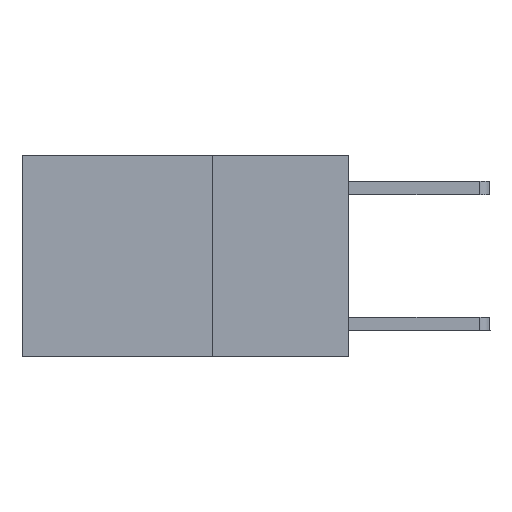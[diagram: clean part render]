
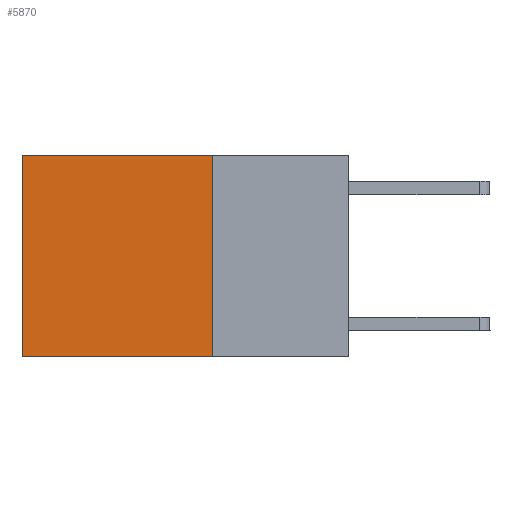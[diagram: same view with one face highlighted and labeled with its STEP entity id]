
A CAD part, left-side view. The second image highlights one B-rep face of the part: STEP entity #5870.
In plain terms, the highlighted planar face has unit normal (-1, 0, 0).
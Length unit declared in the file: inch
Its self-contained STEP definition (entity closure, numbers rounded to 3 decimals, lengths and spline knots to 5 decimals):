
#157 = ORIENTED_EDGE ( 'NONE', *, *, #7674, .F. ) ;
#213 = VERTEX_POINT ( 'NONE', #2378 ) ;
#574 = EDGE_CURVE ( 'NONE', #4029, #8220, #2611, .T. ) ;
#630 = DIRECTION ( 'NONE',  ( 1., 0., 0. ) ) ;
#724 = LINE ( 'NONE', #4210, #4549 ) ;
#750 = VECTOR ( 'NONE', #3371, 39.37008 ) ;
#960 = CARTESIAN_POINT ( 'NONE',  ( 0.2625, 0.25, 0. ) ) ;
#1584 = EDGE_LOOP ( 'NONE', ( #7150, #9272, #157, #9368 ) ) ;
#1886 = CARTESIAN_POINT ( 'NONE',  ( 0.2625, 0.25, -0.37 ) ) ;
#1996 = CARTESIAN_POINT ( 'NONE',  ( 0.2625, 0.25, 0. ) ) ;
#2378 = CARTESIAN_POINT ( 'NONE',  ( 0.2625, 0.25, -0.37 ) ) ;
#2611 = LINE ( 'NONE', #7717, #8080 ) ;
#2726 = VERTEX_POINT ( 'NONE', #6996 ) ;
#2861 = AXIS2_PLACEMENT_3D ( 'NONE', #4437, #630, #5959 ) ;
#3371 = DIRECTION ( 'NONE',  ( 0., 1., 0. ) ) ;
#4010 = FACE_OUTER_BOUND ( 'NONE', #1584, .T. ) ;
#4029 = VERTEX_POINT ( 'NONE', #1996 ) ;
#4210 = CARTESIAN_POINT ( 'NONE',  ( 0.2625, 0.6, 0. ) ) ;
#4437 = CARTESIAN_POINT ( 'NONE',  ( 0.2625, 0.25, 0. ) ) ;
#4549 = VECTOR ( 'NONE', #5732, 39.37008 ) ;
#5732 = DIRECTION ( 'NONE',  ( 0., 0., -1. ) ) ;
#5870 = ADVANCED_FACE ( 'NONE', ( #4010 ), #6619, .F. ) ;
#5959 = DIRECTION ( 'NONE',  ( 0., 0., -1. ) ) ;
#6619 = PLANE ( 'NONE',  #2861 ) ;
#6996 = CARTESIAN_POINT ( 'NONE',  ( 0.2625, 0.6, -0.37 ) ) ;
#7022 = DIRECTION ( 'NONE',  ( 0., 0., -1. ) ) ;
#7028 = LINE ( 'NONE', #1886, #750 ) ;
#7150 = ORIENTED_EDGE ( 'NONE', *, *, #9040, .T. ) ;
#7478 = VECTOR ( 'NONE', #7022, 39.37008 ) ;
#7674 = EDGE_CURVE ( 'NONE', #4029, #213, #9307, .T. ) ;
#7717 = CARTESIAN_POINT ( 'NONE',  ( 0.2625, 0.25, 0. ) ) ;
#7770 = EDGE_CURVE ( 'NONE', #213, #2726, #7028, .T. ) ;
#8080 = VECTOR ( 'NONE', #9316, 39.37008 ) ;
#8220 = VERTEX_POINT ( 'NONE', #9481 ) ;
#9040 = EDGE_CURVE ( 'NONE', #8220, #2726, #724, .T. ) ;
#9272 = ORIENTED_EDGE ( 'NONE', *, *, #7770, .F. ) ;
#9307 = LINE ( 'NONE', #960, #7478 ) ;
#9316 = DIRECTION ( 'NONE',  ( 0., 1., 0. ) ) ;
#9368 = ORIENTED_EDGE ( 'NONE', *, *, #574, .T. ) ;
#9481 = CARTESIAN_POINT ( 'NONE',  ( 0.2625, 0.6, 0. ) ) ;
